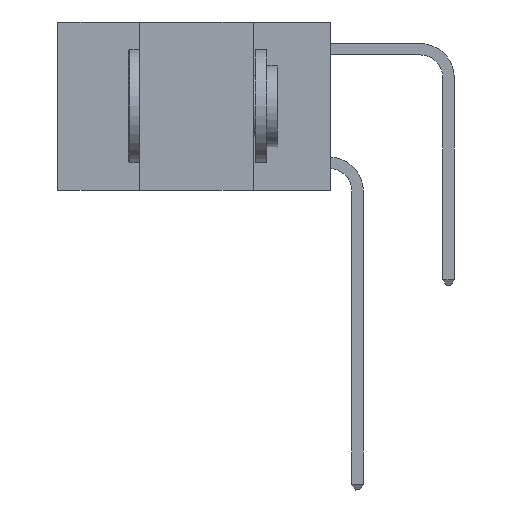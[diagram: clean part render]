
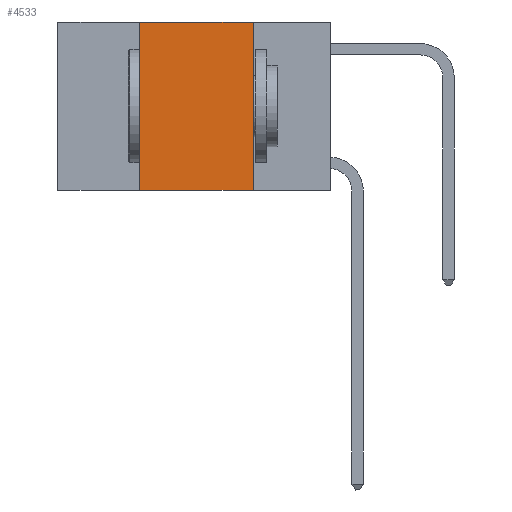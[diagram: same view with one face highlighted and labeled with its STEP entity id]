
A CAD part, left-side view. The second image highlights one B-rep face of the part: STEP entity #4533.
In plain terms, the highlighted planar face has unit normal (-1, 0, 0).
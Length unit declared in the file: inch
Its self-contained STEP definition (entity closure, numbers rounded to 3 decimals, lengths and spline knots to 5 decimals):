
#692 = VECTOR ( 'NONE', #7544, 39.37008 ) ;
#1849 = EDGE_CURVE ( 'NONE', #13738, #12253, #3211, .T. ) ;
#2063 = VECTOR ( 'NONE', #7663, 39.37008 ) ;
#2155 = DIRECTION ( 'NONE',  ( 0., 0., -1. ) ) ;
#2383 = ORIENTED_EDGE ( 'NONE', *, *, #5006, .F. ) ;
#2393 = LINE ( 'NONE', #3031, #692 ) ;
#2729 = CARTESIAN_POINT ( 'NONE',  ( 0., 0.17, 0. ) ) ;
#2767 = CARTESIAN_POINT ( 'NONE',  ( 0., 0.42, 0. ) ) ;
#3031 = CARTESIAN_POINT ( 'NONE',  ( 0., 0.42, 0. ) ) ;
#3211 = LINE ( 'NONE', #2729, #2063 ) ;
#3223 = DIRECTION ( 'NONE',  ( 0., -1., 0. ) ) ;
#4533 = ADVANCED_FACE ( 'NONE', ( #13433 ), #12824, .F. ) ;
#5006 = EDGE_CURVE ( 'NONE', #7938, #13738, #14529, .T. ) ;
#5670 = CARTESIAN_POINT ( 'NONE',  ( 0., 0.6, 0. ) ) ;
#7408 = EDGE_LOOP ( 'NONE', ( #13113, #2383, #12408, #13102 ) ) ;
#7544 = DIRECTION ( 'NONE',  ( 0., 0., 1. ) ) ;
#7663 = DIRECTION ( 'NONE',  ( 0., 0., -1. ) ) ;
#7938 = VERTEX_POINT ( 'NONE', #2767 ) ;
#8867 = VERTEX_POINT ( 'NONE', #14308 ) ;
#9467 = CARTESIAN_POINT ( 'NONE',  ( 0., 0.6, 0. ) ) ;
#9728 = DIRECTION ( 'NONE',  ( 0., -1., 0. ) ) ;
#9969 = EDGE_CURVE ( 'NONE', #8867, #12253, #13367, .T. ) ;
#10647 = CARTESIAN_POINT ( 'NONE',  ( 0., 0.17, -0.37 ) ) ;
#12172 = AXIS2_PLACEMENT_3D ( 'NONE', #9467, #15207, #2155 ) ;
#12253 = VERTEX_POINT ( 'NONE', #10647 ) ;
#12408 = ORIENTED_EDGE ( 'NONE', *, *, #14137, .F. ) ;
#12824 = PLANE ( 'NONE',  #12172 ) ;
#12843 = VECTOR ( 'NONE', #3223, 39.37008 ) ;
#13102 = ORIENTED_EDGE ( 'NONE', *, *, #9969, .T. ) ;
#13113 = ORIENTED_EDGE ( 'NONE', *, *, #1849, .F. ) ;
#13162 = VECTOR ( 'NONE', #9728, 39.37008 ) ;
#13367 = LINE ( 'NONE', #14622, #13162 ) ;
#13433 = FACE_OUTER_BOUND ( 'NONE', #7408, .T. ) ;
#13738 = VERTEX_POINT ( 'NONE', #14331 ) ;
#14137 = EDGE_CURVE ( 'NONE', #8867, #7938, #2393, .T. ) ;
#14308 = CARTESIAN_POINT ( 'NONE',  ( 0., 0.42, -0.37 ) ) ;
#14331 = CARTESIAN_POINT ( 'NONE',  ( 0., 0.17, 0. ) ) ;
#14529 = LINE ( 'NONE', #5670, #12843 ) ;
#14622 = CARTESIAN_POINT ( 'NONE',  ( 0., 0.6, -0.37 ) ) ;
#15207 = DIRECTION ( 'NONE',  ( 1., 0., 0. ) ) ;
